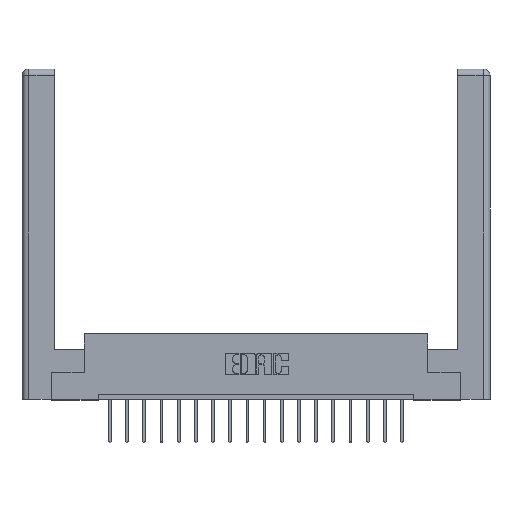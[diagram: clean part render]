
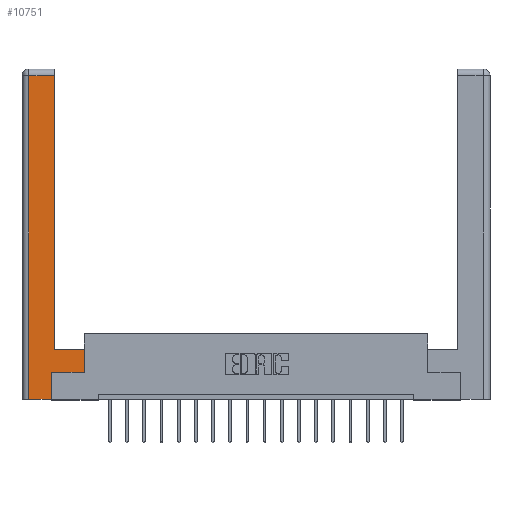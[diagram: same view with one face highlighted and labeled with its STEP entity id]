
A CAD part, top view. The second image highlights one B-rep face of the part: STEP entity #10751.
In plain terms, the highlighted planar face has unit normal (0, 0, 1).
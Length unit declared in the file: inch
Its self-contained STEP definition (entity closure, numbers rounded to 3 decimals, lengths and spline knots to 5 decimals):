
#436 = VERTEX_POINT ( 'NONE', #16600 ) ;
#457 = DIRECTION ( 'NONE',  ( 0., 1., 0. ) ) ;
#506 = LINE ( 'NONE', #17907, #17616 ) ;
#637 = VERTEX_POINT ( 'NONE', #13325 ) ;
#1036 = DIRECTION ( 'NONE',  ( 0., 0., -1. ) ) ;
#1386 = AXIS2_PLACEMENT_3D ( 'NONE', #5580, #1036, #3992 ) ;
#1536 = EDGE_CURVE ( 'NONE', #9319, #436, #506, .T. ) ;
#1739 = VECTOR ( 'NONE', #18206, 39.37008 ) ;
#1776 = CARTESIAN_POINT ( 'NONE',  ( 0.565, 0.45, 0. ) ) ;
#2119 = CARTESIAN_POINT ( 'NONE',  ( 0.565, 0.45, 0. ) ) ;
#2596 = DIRECTION ( 'NONE',  ( 1., 0., 0. ) ) ;
#2659 = VECTOR ( 'NONE', #12750, 39.37008 ) ;
#3148 = DIRECTION ( 'NONE',  ( 0., 1., 0. ) ) ;
#3472 = VECTOR ( 'NONE', #457, 39.37008 ) ;
#3553 = CARTESIAN_POINT ( 'NONE',  ( 0.295, 2.94, 0. ) ) ;
#3587 = VECTOR ( 'NONE', #11938, 39.37008 ) ;
#3842 = ORIENTED_EDGE ( 'NONE', *, *, #14946, .T. ) ;
#3992 = DIRECTION ( 'NONE',  ( -1., 0., 0. ) ) ;
#4015 = VECTOR ( 'NONE', #2596, 39.37008 ) ;
#4554 = VECTOR ( 'NONE', #3148, 39.37008 ) ;
#4787 = LINE ( 'NONE', #1776, #4554 ) ;
#4955 = CARTESIAN_POINT ( 'NONE',  ( 0.565, 0.245, 0. ) ) ;
#5206 = EDGE_CURVE ( 'NONE', #5684, #16218, #8484, .T. ) ;
#5266 = EDGE_CURVE ( 'NONE', #436, #14562, #7562, .T. ) ;
#5288 = EDGE_CURVE ( 'NONE', #14562, #5684, #17700, .T. ) ;
#5441 = PLANE ( 'NONE',  #1386 ) ;
#5508 = EDGE_CURVE ( 'NONE', #637, #8140, #15935, .T. ) ;
#5564 = CARTESIAN_POINT ( 'NONE',  ( 0.0615, 0., 0. ) ) ;
#5580 = CARTESIAN_POINT ( 'NONE',  ( 0., 0., 0. ) ) ;
#5648 = CARTESIAN_POINT ( 'NONE',  ( 0.265, 0.245, 0. ) ) ;
#5684 = VERTEX_POINT ( 'NONE', #18501 ) ;
#5907 = DIRECTION ( 'NONE',  ( -1., 0., 0. ) ) ;
#6231 = ORIENTED_EDGE ( 'NONE', *, *, #5206, .T. ) ;
#6293 = CARTESIAN_POINT ( 'NONE',  ( 0.265, 0.245, 0. ) ) ;
#6590 = EDGE_LOOP ( 'NONE', ( #16856, #8402, #6231, #3842, #15927, #16140, #18250, #14812 ) ) ;
#7428 = EDGE_CURVE ( 'NONE', #8140, #9620, #9190, .T. ) ;
#7562 = LINE ( 'NONE', #14696, #3587 ) ;
#7746 = VECTOR ( 'NONE', #5907, 39.37008 ) ;
#8140 = VERTEX_POINT ( 'NONE', #5648 ) ;
#8259 = CARTESIAN_POINT ( 'NONE',  ( 0.265, 0., 0. ) ) ;
#8402 = ORIENTED_EDGE ( 'NONE', *, *, #5288, .T. ) ;
#8484 = LINE ( 'NONE', #5564, #2659 ) ;
#8755 = CARTESIAN_POINT ( 'NONE',  ( 0.0615, 2.94, 0. ) ) ;
#8860 = FACE_OUTER_BOUND ( 'NONE', #6590, .T. ) ;
#9190 = LINE ( 'NONE', #4955, #1739 ) ;
#9319 = VERTEX_POINT ( 'NONE', #2119 ) ;
#9620 = VERTEX_POINT ( 'NONE', #13411 ) ;
#9622 = CARTESIAN_POINT ( 'NONE',  ( 0.0615, 0., 0. ) ) ;
#10563 = DIRECTION ( 'NONE',  ( -1., 0., 0. ) ) ;
#10751 = ADVANCED_FACE ( 'NONE', ( #8860 ), #5441, .F. ) ;
#11938 = DIRECTION ( 'NONE',  ( 0., 1., 0. ) ) ;
#12750 = DIRECTION ( 'NONE',  ( 0., -1., 0. ) ) ;
#13325 = CARTESIAN_POINT ( 'NONE',  ( 0.265, 0., 0. ) ) ;
#13411 = CARTESIAN_POINT ( 'NONE',  ( 0.565, 0.245, 0. ) ) ;
#14562 = VERTEX_POINT ( 'NONE', #3553 ) ;
#14696 = CARTESIAN_POINT ( 'NONE',  ( 0.295, 3., 0. ) ) ;
#14812 = ORIENTED_EDGE ( 'NONE', *, *, #1536, .T. ) ;
#14946 = EDGE_CURVE ( 'NONE', #16218, #637, #17645, .T. ) ;
#15927 = ORIENTED_EDGE ( 'NONE', *, *, #5508, .T. ) ;
#15935 = LINE ( 'NONE', #6293, #3472 ) ;
#16140 = ORIENTED_EDGE ( 'NONE', *, *, #7428, .T. ) ;
#16218 = VERTEX_POINT ( 'NONE', #9622 ) ;
#16600 = CARTESIAN_POINT ( 'NONE',  ( 0.295, 0.45, 0. ) ) ;
#16856 = ORIENTED_EDGE ( 'NONE', *, *, #5266, .T. ) ;
#17616 = VECTOR ( 'NONE', #10563, 39.37008 ) ;
#17645 = LINE ( 'NONE', #8259, #4015 ) ;
#17700 = LINE ( 'NONE', #8755, #7746 ) ;
#17907 = CARTESIAN_POINT ( 'NONE',  ( 0.295, 0.45, 0. ) ) ;
#18206 = DIRECTION ( 'NONE',  ( 1., 0., 0. ) ) ;
#18250 = ORIENTED_EDGE ( 'NONE', *, *, #19128, .T. ) ;
#18501 = CARTESIAN_POINT ( 'NONE',  ( 0.0615, 2.94, 0. ) ) ;
#19128 = EDGE_CURVE ( 'NONE', #9620, #9319, #4787, .T. ) ;
